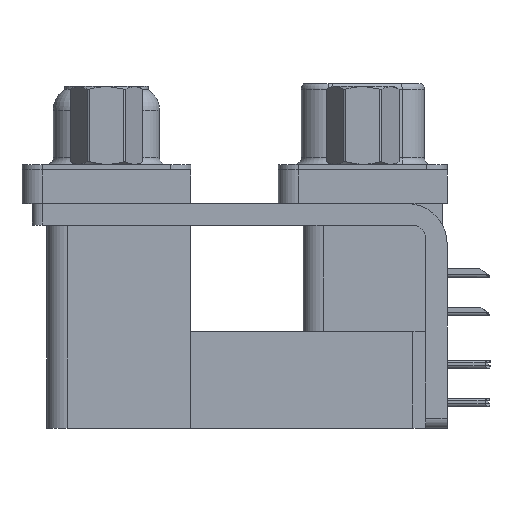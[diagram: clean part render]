
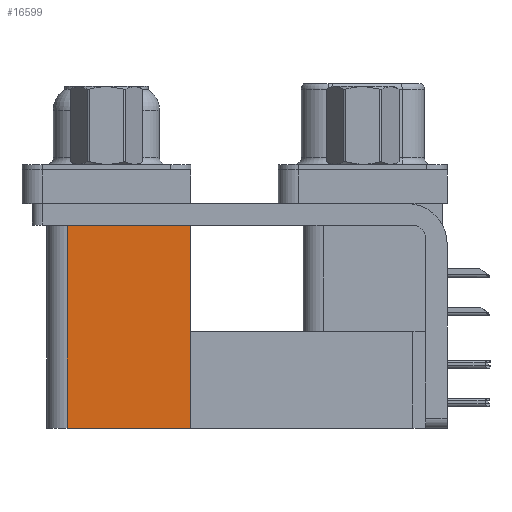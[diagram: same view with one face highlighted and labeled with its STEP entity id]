
A CAD part, left-side view. The second image highlights one B-rep face of the part: STEP entity #16599.
In plain terms, the highlighted planar face has unit normal (-1, 0, 0).
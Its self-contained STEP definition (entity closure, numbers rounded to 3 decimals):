
#119 = VECTOR ( 'NONE', #48814, 1000. ) ;
#229 = DIRECTION ( 'NONE',  ( 0., 1., 0. ) ) ;
#510 = ORIENTED_EDGE ( 'NONE', *, *, #43402, .T. ) ;
#3347 = EDGE_CURVE ( 'NONE', #17636, #40313, #34698, .T. ) ;
#4651 = EDGE_LOOP ( 'NONE', ( #510, #26325, #42265, #41649 ) ) ;
#7597 = CARTESIAN_POINT ( 'NONE',  ( 3.765, 21.975, -19.2 ) ) ;
#8627 = AXIS2_PLACEMENT_3D ( 'NONE', #12325, #38497, #229 ) ;
#11004 = VERTEX_POINT ( 'NONE', #34502 ) ;
#12325 = CARTESIAN_POINT ( 'NONE',  ( 3.765, 12.775, -19.2 ) ) ;
#12383 = CARTESIAN_POINT ( 'NONE',  ( 3.765, 12.775, -19.2 ) ) ;
#14966 = CARTESIAN_POINT ( 'NONE',  ( 3.765, 12.775, -2.5 ) ) ;
#16313 = LINE ( 'NONE', #27660, #42853 ) ;
#16599 = ADVANCED_FACE ( 'NONE', ( #19712 ), #41487, .F. ) ;
#17636 = VERTEX_POINT ( 'NONE', #12383 ) ;
#18525 = EDGE_CURVE ( 'NONE', #11004, #43520, #34499, .T. ) ;
#19712 = FACE_OUTER_BOUND ( 'NONE', #4651, .T. ) ;
#21490 = CARTESIAN_POINT ( 'NONE',  ( 3.765, 21.975, -2.5 ) ) ;
#22285 = VECTOR ( 'NONE', #33585, 1000. ) ;
#22904 = DIRECTION ( 'NONE',  ( 0., 0., 1. ) ) ;
#24995 = VECTOR ( 'NONE', #22904, 1000. ) ;
#26325 = ORIENTED_EDGE ( 'NONE', *, *, #18525, .F. ) ;
#27660 = CARTESIAN_POINT ( 'NONE',  ( 3.765, 12.775, -2.5 ) ) ;
#29962 = EDGE_CURVE ( 'NONE', #17636, #11004, #34317, .T. ) ;
#30821 = CARTESIAN_POINT ( 'NONE',  ( 3.765, 12.775, -19.2 ) ) ;
#31368 = DIRECTION ( 'NONE',  ( 0., 1., 0. ) ) ;
#33585 = DIRECTION ( 'NONE',  ( 0., 1., 0. ) ) ;
#34317 = LINE ( 'NONE', #30821, #22285 ) ;
#34499 = LINE ( 'NONE', #7597, #24995 ) ;
#34502 = CARTESIAN_POINT ( 'NONE',  ( 3.765, 21.975, -19.2 ) ) ;
#34698 = LINE ( 'NONE', #38186, #119 ) ;
#38186 = CARTESIAN_POINT ( 'NONE',  ( 3.765, 12.775, -19.2 ) ) ;
#38497 = DIRECTION ( 'NONE',  ( 1., 0., 0. ) ) ;
#40313 = VERTEX_POINT ( 'NONE', #14966 ) ;
#41487 = PLANE ( 'NONE',  #8627 ) ;
#41649 = ORIENTED_EDGE ( 'NONE', *, *, #3347, .T. ) ;
#42265 = ORIENTED_EDGE ( 'NONE', *, *, #29962, .F. ) ;
#42853 = VECTOR ( 'NONE', #31368, 1000. ) ;
#43402 = EDGE_CURVE ( 'NONE', #40313, #43520, #16313, .T. ) ;
#43520 = VERTEX_POINT ( 'NONE', #21490 ) ;
#48814 = DIRECTION ( 'NONE',  ( 0., 0., 1. ) ) ;
